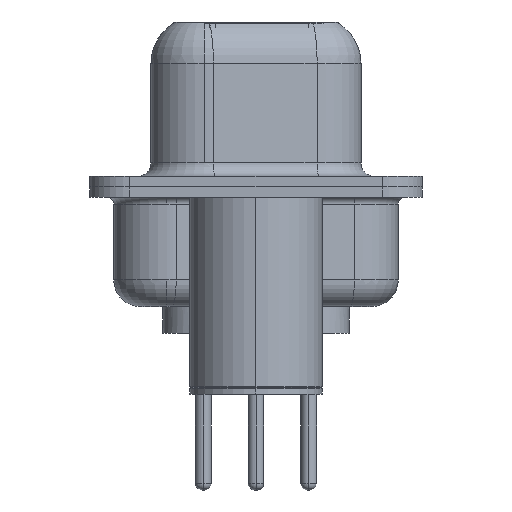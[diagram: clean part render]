
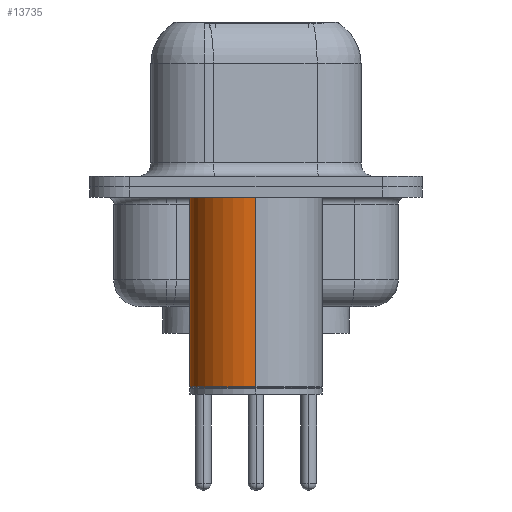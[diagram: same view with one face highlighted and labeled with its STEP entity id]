
A CAD part, left-side view. The second image highlights one B-rep face of the part: STEP entity #13735.
In plain terms, the highlighted cylindrical face has radius 2.5 mm (diameter 5 mm), a partial arc.
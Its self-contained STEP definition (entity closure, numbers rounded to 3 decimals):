
#154 = DIRECTION ( 'NONE',  ( 0., 0., 1. ) ) ;
#567 = LINE ( 'NONE', #10211, #13447 ) ;
#1619 = VERTEX_POINT ( 'NONE', #16475 ) ;
#1991 = VERTEX_POINT ( 'NONE', #28305 ) ;
#2225 = CARTESIAN_POINT ( 'NONE',  ( 0., 0., -0.4 ) ) ;
#2637 = DIRECTION ( 'NONE',  ( 0., 0., 1. ) ) ;
#2967 = EDGE_CURVE ( 'NONE', #1991, #12240, #30365, .T. ) ;
#3347 = CIRCLE ( 'NONE', #27112, 2.5 ) ;
#3635 = ORIENTED_EDGE ( 'NONE', *, *, #17778, .F. ) ;
#5833 = DIRECTION ( 'NONE',  ( 0., 0., 1. ) ) ;
#6167 = EDGE_CURVE ( 'NONE', #23684, #1991, #23745, .T. ) ;
#6574 = EDGE_CURVE ( 'NONE', #23684, #1619, #567, .T. ) ;
#8156 = VECTOR ( 'NONE', #5833, 1000. ) ;
#10211 = CARTESIAN_POINT ( 'NONE',  ( 2.5, 0., 0.581 ) ) ;
#10400 = DIRECTION ( 'NONE',  ( 1., 0., 0. ) ) ;
#11350 = CARTESIAN_POINT ( 'NONE',  ( -2.5, 0., 0.581 ) ) ;
#12240 = VERTEX_POINT ( 'NONE', #25791 ) ;
#13447 = VECTOR ( 'NONE', #2637, 1000. ) ;
#13720 = AXIS2_PLACEMENT_3D ( 'NONE', #30054, #27353, #24840 ) ;
#13735 = ADVANCED_FACE ( 'NONE', ( #19466 ), #29288, .T. ) ;
#14990 = CARTESIAN_POINT ( 'NONE',  ( 0., 0., -7.525 ) ) ;
#15869 = EDGE_LOOP ( 'NONE', ( #25981, #22119, #3635, #20832 ) ) ;
#16475 = CARTESIAN_POINT ( 'NONE',  ( 2.5, 0., -0.4 ) ) ;
#17778 = EDGE_CURVE ( 'NONE', #1619, #12240, #3347, .T. ) ;
#19466 = FACE_OUTER_BOUND ( 'NONE', #15869, .T. ) ;
#19702 = CARTESIAN_POINT ( 'NONE',  ( 2.5, 0., -7.525 ) ) ;
#20832 = ORIENTED_EDGE ( 'NONE', *, *, #6574, .F. ) ;
#22119 = ORIENTED_EDGE ( 'NONE', *, *, #2967, .T. ) ;
#22137 = DIRECTION ( 'NONE',  ( 0., 0., 1. ) ) ;
#23237 = AXIS2_PLACEMENT_3D ( 'NONE', #14990, #22137, #10400 ) ;
#23684 = VERTEX_POINT ( 'NONE', #19702 ) ;
#23745 = CIRCLE ( 'NONE', #23237, 2.5 ) ;
#24840 = DIRECTION ( 'NONE',  ( 1., 0., 0. ) ) ;
#25791 = CARTESIAN_POINT ( 'NONE',  ( -2.5, 0., -0.4 ) ) ;
#25981 = ORIENTED_EDGE ( 'NONE', *, *, #6167, .T. ) ;
#27112 = AXIS2_PLACEMENT_3D ( 'NONE', #2225, #154, #31198 ) ;
#27353 = DIRECTION ( 'NONE',  ( 0., 0., 1. ) ) ;
#28305 = CARTESIAN_POINT ( 'NONE',  ( -2.5, 0., -7.525 ) ) ;
#29288 = CYLINDRICAL_SURFACE ( 'NONE', #13720, 2.5 ) ;
#30054 = CARTESIAN_POINT ( 'NONE',  ( 0., 0., 0.581 ) ) ;
#30365 = LINE ( 'NONE', #11350, #8156 ) ;
#31198 = DIRECTION ( 'NONE',  ( 1., 0., 0. ) ) ;
